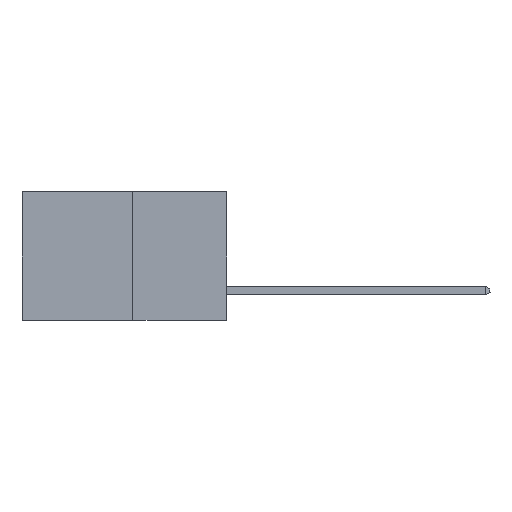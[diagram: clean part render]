
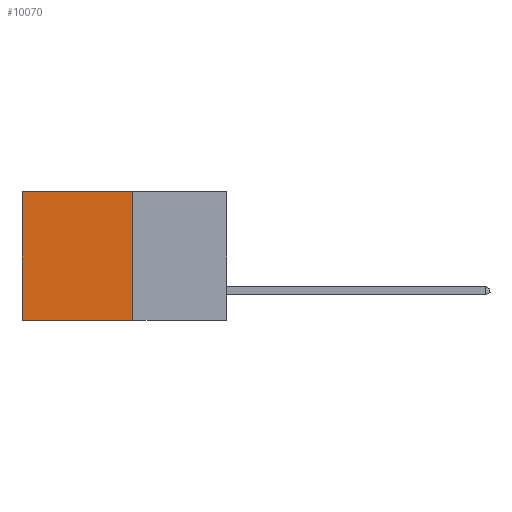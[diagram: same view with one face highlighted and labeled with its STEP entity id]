
A CAD part, left-side view. The second image highlights one B-rep face of the part: STEP entity #10070.
In plain terms, the highlighted planar face has unit normal (-1, 0, 0).
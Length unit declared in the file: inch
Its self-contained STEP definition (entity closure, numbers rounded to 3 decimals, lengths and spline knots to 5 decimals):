
#313 = CARTESIAN_POINT ( 'NONE',  ( 0.277, 0.27, -0.37 ) ) ;
#386 = DIRECTION ( 'NONE',  ( 0., 1., 0. ) ) ;
#393 = VERTEX_POINT ( 'NONE', #2338 ) ;
#471 = LINE ( 'NONE', #604, #11010 ) ;
#545 = EDGE_CURVE ( 'NONE', #9496, #9419, #4212, .T. ) ;
#551 = DIRECTION ( 'NONE',  ( 0., 1., 0. ) ) ;
#604 = CARTESIAN_POINT ( 'NONE',  ( 0.277, 0.27, 0. ) ) ;
#1205 = ORIENTED_EDGE ( 'NONE', *, *, #1253, .T. ) ;
#1253 = EDGE_CURVE ( 'NONE', #12098, #9419, #4830, .T. ) ;
#1524 = CARTESIAN_POINT ( 'NONE',  ( 0.277, 0.59, -0.37 ) ) ;
#1874 = EDGE_LOOP ( 'NONE', ( #1205, #9240, #9323, #7563 ) ) ;
#2209 = EDGE_CURVE ( 'NONE', #393, #12098, #471, .T. ) ;
#2338 = CARTESIAN_POINT ( 'NONE',  ( 0.277, 0.27, 0. ) ) ;
#2542 = EDGE_CURVE ( 'NONE', #393, #9496, #8284, .T. ) ;
#4212 = LINE ( 'NONE', #11880, #11651 ) ;
#4615 = DIRECTION ( 'NONE',  ( 1., 0., 0. ) ) ;
#4830 = LINE ( 'NONE', #9113, #9998 ) ;
#6765 = CARTESIAN_POINT ( 'NONE',  ( 0.277, 0.27, -0.37 ) ) ;
#7563 = ORIENTED_EDGE ( 'NONE', *, *, #2209, .T. ) ;
#7742 = CARTESIAN_POINT ( 'NONE',  ( 0.277, 0.59, 0. ) ) ;
#7957 = VECTOR ( 'NONE', #8640, 39.37008 ) ;
#8218 = CARTESIAN_POINT ( 'NONE',  ( 0.277, 0.27, -0.37 ) ) ;
#8284 = LINE ( 'NONE', #313, #7957 ) ;
#8304 = FACE_OUTER_BOUND ( 'NONE', #1874, .T. ) ;
#8640 = DIRECTION ( 'NONE',  ( 0., 0., -1. ) ) ;
#9113 = CARTESIAN_POINT ( 'NONE',  ( 0.277, 0.59, -0.37 ) ) ;
#9240 = ORIENTED_EDGE ( 'NONE', *, *, #545, .F. ) ;
#9323 = ORIENTED_EDGE ( 'NONE', *, *, #2542, .F. ) ;
#9419 = VERTEX_POINT ( 'NONE', #1524 ) ;
#9496 = VERTEX_POINT ( 'NONE', #8218 ) ;
#9998 = VECTOR ( 'NONE', #11113, 39.37008 ) ;
#10070 = ADVANCED_FACE ( 'NONE', ( #8304 ), #13350, .F. ) ;
#11010 = VECTOR ( 'NONE', #551, 39.37008 ) ;
#11113 = DIRECTION ( 'NONE',  ( 0., 0., -1. ) ) ;
#11642 = DIRECTION ( 'NONE',  ( 0., 0., -1. ) ) ;
#11651 = VECTOR ( 'NONE', #386, 39.37008 ) ;
#11880 = CARTESIAN_POINT ( 'NONE',  ( 0.277, 0.27, -0.37 ) ) ;
#12098 = VERTEX_POINT ( 'NONE', #7742 ) ;
#12609 = AXIS2_PLACEMENT_3D ( 'NONE', #6765, #4615, #11642 ) ;
#13350 = PLANE ( 'NONE',  #12609 ) ;
